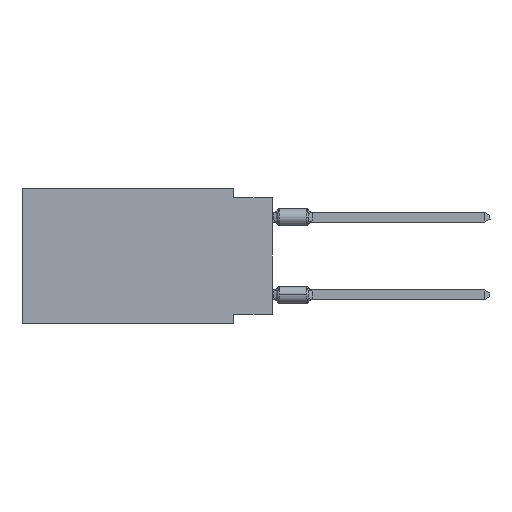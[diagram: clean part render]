
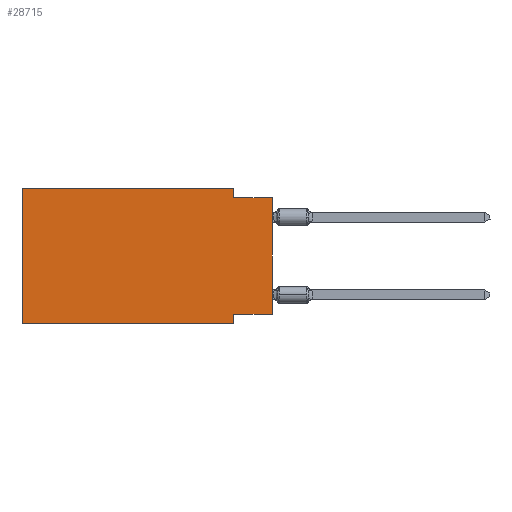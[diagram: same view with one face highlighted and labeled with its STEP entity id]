
A CAD part, left-side view. The second image highlights one B-rep face of the part: STEP entity #28715.
In plain terms, the highlighted planar face has unit normal (-1, 0, 0).
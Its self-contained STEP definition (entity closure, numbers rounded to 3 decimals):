
#368 = DIRECTION ( 'NONE',  ( 0., 0., -1. ) ) ;
#1023 = CARTESIAN_POINT ( 'NONE',  ( 0., 16.383, 0. ) ) ;
#1559 = EDGE_CURVE ( 'NONE', #45711, #15176, #27989, .T. ) ;
#2524 = VECTOR ( 'NONE', #368, 1000. ) ;
#3021 = VERTEX_POINT ( 'NONE', #55317 ) ;
#3356 = DIRECTION ( 'NONE',  ( 0., 0., 1. ) ) ;
#4960 = LINE ( 'NONE', #39986, #2524 ) ;
#6499 = FACE_OUTER_BOUND ( 'NONE', #42370, .T. ) ;
#6690 = VECTOR ( 'NONE', #10211, 1000. ) ;
#6776 = DIRECTION ( 'NONE',  ( 0., 0., -1. ) ) ;
#9651 = LINE ( 'NONE', #36323, #25897 ) ;
#10211 = DIRECTION ( 'NONE',  ( 0., -1., 0. ) ) ;
#11254 = EDGE_CURVE ( 'NONE', #56176, #45711, #11985, .T. ) ;
#11985 = LINE ( 'NONE', #43530, #33054 ) ;
#12746 = EDGE_CURVE ( 'NONE', #25609, #3021, #9651, .T. ) ;
#15176 = VERTEX_POINT ( 'NONE', #46739 ) ;
#15708 = CARTESIAN_POINT ( 'NONE',  ( 0., 2.54, -8.255 ) ) ;
#16654 = CARTESIAN_POINT ( 'NONE',  ( 0., 16.383, -8.89 ) ) ;
#19665 = PLANE ( 'NONE',  #27185 ) ;
#19715 = EDGE_CURVE ( 'NONE', #47432, #53111, #43255, .T. ) ;
#21113 = CARTESIAN_POINT ( 'NONE',  ( 0., 2.54, -8.89 ) ) ;
#25282 = ORIENTED_EDGE ( 'NONE', *, *, #12746, .F. ) ;
#25609 = VERTEX_POINT ( 'NONE', #47524 ) ;
#25897 = VECTOR ( 'NONE', #44968, 1000. ) ;
#27040 = ORIENTED_EDGE ( 'NONE', *, *, #11254, .F. ) ;
#27185 = AXIS2_PLACEMENT_3D ( 'NONE', #54754, #50452, #6776 ) ;
#27960 = LINE ( 'NONE', #32854, #47990 ) ;
#27989 = LINE ( 'NONE', #1023, #6690 ) ;
#28715 = ADVANCED_FACE ( 'NONE', ( #6499 ), #19665, .F. ) ;
#28929 = VECTOR ( 'NONE', #32326, 1000. ) ;
#29661 = CARTESIAN_POINT ( 'NONE',  ( 0., 0., 0. ) ) ;
#32154 = EDGE_CURVE ( 'NONE', #47432, #3021, #37179, .T. ) ;
#32326 = DIRECTION ( 'NONE',  ( 0., 0., 1. ) ) ;
#32339 = ORIENTED_EDGE ( 'NONE', *, *, #53529, .F. ) ;
#32474 = ORIENTED_EDGE ( 'NONE', *, *, #1559, .F. ) ;
#32854 = CARTESIAN_POINT ( 'NONE',  ( 0., 2.54, -8.89 ) ) ;
#33054 = VECTOR ( 'NONE', #3356, 1000. ) ;
#34157 = EDGE_CURVE ( 'NONE', #15176, #25609, #4960, .T. ) ;
#35012 = LINE ( 'NONE', #16654, #47841 ) ;
#36323 = CARTESIAN_POINT ( 'NONE',  ( 0., 0., -0.635 ) ) ;
#36660 = VECTOR ( 'NONE', #46736, 1000. ) ;
#37179 = LINE ( 'NONE', #29661, #28929 ) ;
#39986 = CARTESIAN_POINT ( 'NONE',  ( 0., 2.54, 0. ) ) ;
#40645 = CARTESIAN_POINT ( 'NONE',  ( 0., 0., -8.255 ) ) ;
#41353 = EDGE_CURVE ( 'NONE', #56176, #51990, #35012, .T. ) ;
#42370 = EDGE_LOOP ( 'NONE', ( #43895, #25282, #52521, #32474, #27040, #44911, #32339, #53595 ) ) ;
#42503 = CARTESIAN_POINT ( 'NONE',  ( 0., 16.383, 0. ) ) ;
#43255 = LINE ( 'NONE', #51336, #36660 ) ;
#43530 = CARTESIAN_POINT ( 'NONE',  ( 0., 16.383, 0. ) ) ;
#43895 = ORIENTED_EDGE ( 'NONE', *, *, #32154, .T. ) ;
#44484 = CARTESIAN_POINT ( 'NONE',  ( 0., 16.383, -8.89 ) ) ;
#44911 = ORIENTED_EDGE ( 'NONE', *, *, #41353, .T. ) ;
#44968 = DIRECTION ( 'NONE',  ( 0., -1., 0. ) ) ;
#45711 = VERTEX_POINT ( 'NONE', #42503 ) ;
#46736 = DIRECTION ( 'NONE',  ( 0., 1., 0. ) ) ;
#46739 = CARTESIAN_POINT ( 'NONE',  ( 0., 2.54, 0. ) ) ;
#47099 = DIRECTION ( 'NONE',  ( 0., -1., 0. ) ) ;
#47432 = VERTEX_POINT ( 'NONE', #40645 ) ;
#47524 = CARTESIAN_POINT ( 'NONE',  ( 0., 2.54, -0.635 ) ) ;
#47841 = VECTOR ( 'NONE', #47099, 1000. ) ;
#47990 = VECTOR ( 'NONE', #54994, 1000. ) ;
#50452 = DIRECTION ( 'NONE',  ( 1., 0., 0. ) ) ;
#51336 = CARTESIAN_POINT ( 'NONE',  ( 0., 0., -8.255 ) ) ;
#51990 = VERTEX_POINT ( 'NONE', #21113 ) ;
#52521 = ORIENTED_EDGE ( 'NONE', *, *, #34157, .F. ) ;
#53111 = VERTEX_POINT ( 'NONE', #15708 ) ;
#53529 = EDGE_CURVE ( 'NONE', #53111, #51990, #27960, .T. ) ;
#53595 = ORIENTED_EDGE ( 'NONE', *, *, #19715, .F. ) ;
#54754 = CARTESIAN_POINT ( 'NONE',  ( 0., 16.383, 0. ) ) ;
#54994 = DIRECTION ( 'NONE',  ( 0., 0., -1. ) ) ;
#55317 = CARTESIAN_POINT ( 'NONE',  ( 0., 0., -0.635 ) ) ;
#56176 = VERTEX_POINT ( 'NONE', #44484 ) ;
